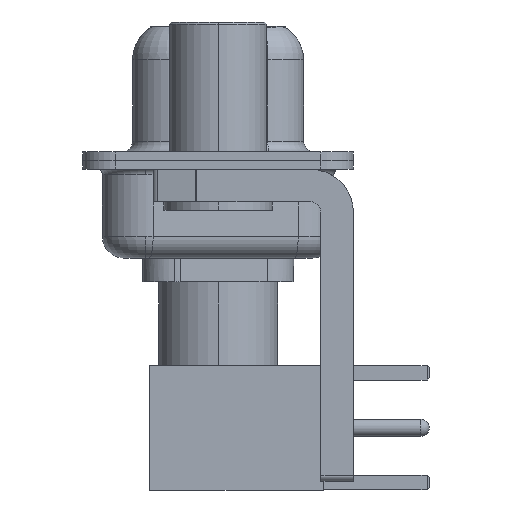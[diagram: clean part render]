
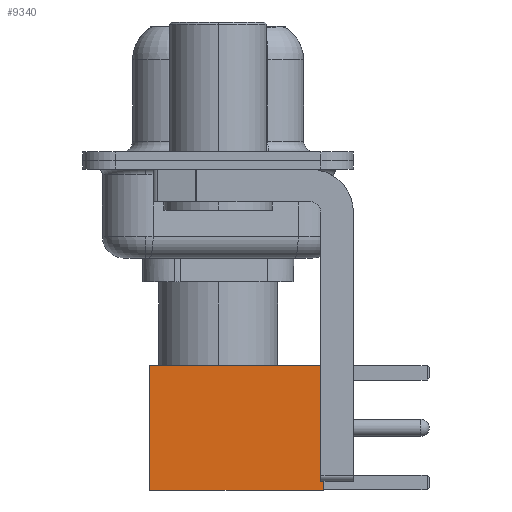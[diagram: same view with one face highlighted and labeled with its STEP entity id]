
A CAD part, left-side view. The second image highlights one B-rep face of the part: STEP entity #9340.
In plain terms, the highlighted face is planar.
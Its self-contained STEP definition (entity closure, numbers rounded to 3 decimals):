
#74 = DIRECTION ( 'NONE',  ( 0., 0., -1. ) ) ;
#545 = VECTOR ( 'NONE', #74, 1000. ) ;
#1433 = LINE ( 'NONE', #10491, #19078 ) ;
#1992 = EDGE_CURVE ( 'NONE', #2992, #9919, #18119, .T. ) ;
#2541 = ORIENTED_EDGE ( 'NONE', *, *, #3982, .T. ) ;
#2608 = CARTESIAN_POINT ( 'NONE',  ( 2.875, 2.875, 0. ) ) ;
#2731 = VECTOR ( 'NONE', #13977, 1000. ) ;
#2992 = VERTEX_POINT ( 'NONE', #3399 ) ;
#3399 = CARTESIAN_POINT ( 'NONE',  ( 2.875, 2.875, 8. ) ) ;
#3420 = CARTESIAN_POINT ( 'NONE',  ( 0., 2.875, 8. ) ) ;
#3427 = LINE ( 'NONE', #12782, #2731 ) ;
#3540 = ORIENTED_EDGE ( 'NONE', *, *, #1992, .T. ) ;
#3982 = EDGE_CURVE ( 'NONE', #9919, #10816, #3427, .T. ) ;
#4059 = VECTOR ( 'NONE', #15448, 1000. ) ;
#4799 = CARTESIAN_POINT ( 'NONE',  ( 2.875, 2.875, 0. ) ) ;
#5307 = ORIENTED_EDGE ( 'NONE', *, *, #15443, .F. ) ;
#6180 = VERTEX_POINT ( 'NONE', #14634 ) ;
#8299 = EDGE_CURVE ( 'NONE', #2992, #6180, #9025, .T. ) ;
#8600 = DIRECTION ( 'NONE',  ( 0., 1., 0. ) ) ;
#8893 = ORIENTED_EDGE ( 'NONE', *, *, #8299, .F. ) ;
#9025 = LINE ( 'NONE', #3420, #4059 ) ;
#9340 = ADVANCED_FACE ( 'NONE', ( #11755 ), #16211, .T. ) ;
#9919 = VERTEX_POINT ( 'NONE', #11136 ) ;
#10491 = CARTESIAN_POINT ( 'NONE',  ( -2.875, 2.875, 0. ) ) ;
#10816 = VERTEX_POINT ( 'NONE', #14355 ) ;
#11136 = CARTESIAN_POINT ( 'NONE',  ( 2.875, 2.875, 0. ) ) ;
#11755 = FACE_OUTER_BOUND ( 'NONE', #15898, .T. ) ;
#11984 = DIRECTION ( 'NONE',  ( 0., 0., -1. ) ) ;
#12782 = CARTESIAN_POINT ( 'NONE',  ( 0., 2.875, 0. ) ) ;
#13347 = DIRECTION ( 'NONE',  ( 0., 0., 1. ) ) ;
#13977 = DIRECTION ( 'NONE',  ( -1., 0., 0. ) ) ;
#14355 = CARTESIAN_POINT ( 'NONE',  ( -2.875, 2.875, 0. ) ) ;
#14634 = CARTESIAN_POINT ( 'NONE',  ( -2.875, 2.875, 8. ) ) ;
#15443 = EDGE_CURVE ( 'NONE', #6180, #10816, #1433, .T. ) ;
#15448 = DIRECTION ( 'NONE',  ( -1., 0., 0. ) ) ;
#15898 = EDGE_LOOP ( 'NONE', ( #3540, #2541, #5307, #8893 ) ) ;
#16211 = PLANE ( 'NONE',  #18063 ) ;
#18063 = AXIS2_PLACEMENT_3D ( 'NONE', #2608, #8600, #13347 ) ;
#18119 = LINE ( 'NONE', #4799, #545 ) ;
#19078 = VECTOR ( 'NONE', #11984, 1000. ) ;
